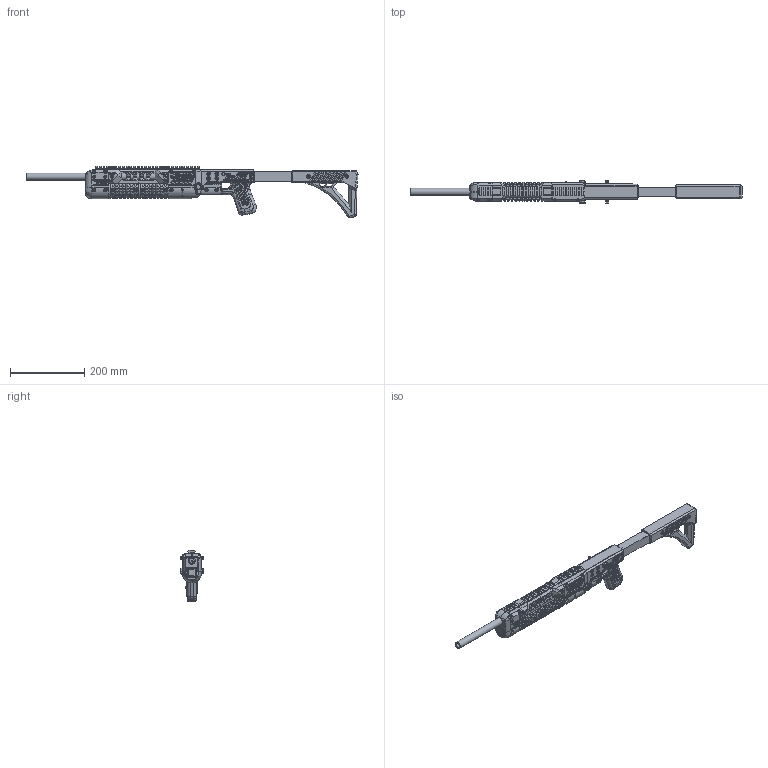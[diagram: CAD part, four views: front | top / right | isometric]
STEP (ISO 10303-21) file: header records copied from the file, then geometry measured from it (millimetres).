
FILE_DESCRIPTION(/* description */ (''),/* implementation_level */ '2;1');
FILE_NAME(/* name */ 'ChimeraV1.4.stp',/* time_stamp */ '2021-03-01T11:02:48-06:00',/* author */ (''),/* organization */ (''),/* preprocessor_version */ 'ST-DEVELOPER v15.2',/* originating_system */ 'Autodesk Translator Framework v2.0.0.5431',/* authorisation */ '');
FILE_SCHEMA (('AUTOMOTIVE_DESIGN { 1 0 10303 214 3 1 1 }'));
Products named in the file (1): ChimeraV1.4
Bounding box: 896.87 x 63.53 x 137.94 mm (x, y, z)
Volume: 1580719 mm3; surface area: 619757.2 mm2
Topology: 90 solids, 90 shells, 4153 faces, 10651 edges, 6906 vertices
Faces by surface type: plane 2475, cylinder 778, bspline 448, cone 248, torus 196, sphere 8
Full cylindrical faces by diameter (mm): 2 x3, 2.1 x1, 2.76 x18, 2.8 x4, 2.85 x1, 2.9 x1, 3 x9, 3.1 x3, 3.125 x16, 3.25 x2, 3.7 x1, 3.8 x12, 3.9 x2, 4.2 x14, 4.6 x38, 4.7 x19, 4.8 x18, 5 x42, 5.1 x58, 6 x8, 6.1 x2, 6.2 x5, 6.3 x4, 6.35 x2, 6.45 x2, 6.85 x2, 7.3 x1, 10 x74, 12.7 x1, 19.05 x1
Entity records: 143344 total; most frequent: CARTESIAN_POINT 47009, ORIENTED_EDGE 19816, DIRECTION 18287, EDGE_CURVE 9908, VERTEX_POINT 6842, LINE 6363, VECTOR 6363, AXIS2_PLACEMENT_3D 5962
